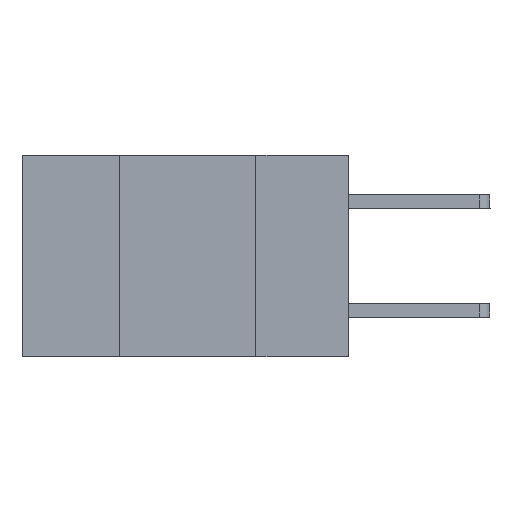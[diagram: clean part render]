
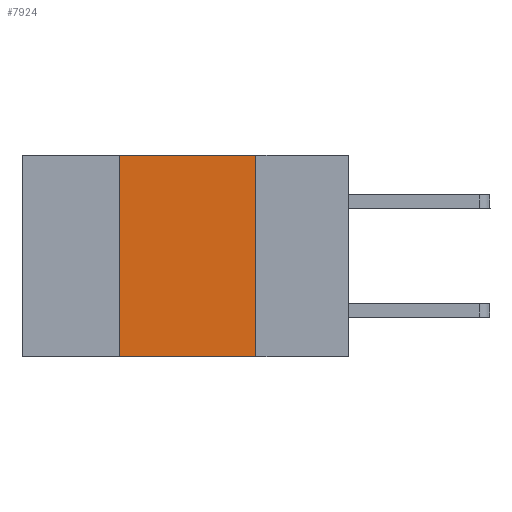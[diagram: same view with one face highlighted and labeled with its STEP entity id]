
A CAD part, left-side view. The second image highlights one B-rep face of the part: STEP entity #7924.
In plain terms, the highlighted planar face has unit normal (-1, 0, 0).
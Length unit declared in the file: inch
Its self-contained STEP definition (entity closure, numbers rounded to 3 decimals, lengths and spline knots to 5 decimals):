
#301 = DIRECTION ( 'NONE',  ( 1., 0., 0. ) ) ;
#354 = VERTEX_POINT ( 'NONE', #8715 ) ;
#697 = CARTESIAN_POINT ( 'NONE',  ( 0., 0.42, 0. ) ) ;
#1254 = PLANE ( 'NONE',  #8034 ) ;
#1422 = EDGE_CURVE ( 'NONE', #5762, #354, #6210, .T. ) ;
#1621 = EDGE_CURVE ( 'NONE', #354, #4686, #5054, .T. ) ;
#1622 = EDGE_CURVE ( 'NONE', #3400, #5762, #7652, .T. ) ;
#1808 = CARTESIAN_POINT ( 'NONE',  ( 0., 0.42, -0.37 ) ) ;
#1980 = CARTESIAN_POINT ( 'NONE',  ( 0., 0.17, -0.37 ) ) ;
#2040 = CARTESIAN_POINT ( 'NONE',  ( 0., 0.42, -0.37 ) ) ;
#2447 = DIRECTION ( 'NONE',  ( 0., -1., 0. ) ) ;
#2830 = VECTOR ( 'NONE', #9318, 39.37008 ) ;
#3367 = DIRECTION ( 'NONE',  ( 0., -1., 0. ) ) ;
#3400 = VERTEX_POINT ( 'NONE', #1808 ) ;
#4135 = VECTOR ( 'NONE', #6768, 39.37008 ) ;
#4367 = ORIENTED_EDGE ( 'NONE', *, *, #1422, .F. ) ;
#4686 = VERTEX_POINT ( 'NONE', #9959 ) ;
#4748 = EDGE_LOOP ( 'NONE', ( #9865, #4367, #9380, #6096 ) ) ;
#5054 = LINE ( 'NONE', #1980, #2830 ) ;
#5762 = VERTEX_POINT ( 'NONE', #697 ) ;
#5933 = FACE_OUTER_BOUND ( 'NONE', #4748, .T. ) ;
#6096 = ORIENTED_EDGE ( 'NONE', *, *, #7256, .T. ) ;
#6210 = LINE ( 'NONE', #6365, #8128 ) ;
#6365 = CARTESIAN_POINT ( 'NONE',  ( 0., 0.6, 0. ) ) ;
#6768 = DIRECTION ( 'NONE',  ( 0., 0., 1. ) ) ;
#7104 = CARTESIAN_POINT ( 'NONE',  ( 0., 0.6, -0.37 ) ) ;
#7256 = EDGE_CURVE ( 'NONE', #3400, #4686, #8100, .T. ) ;
#7652 = LINE ( 'NONE', #2040, #4135 ) ;
#7784 = VECTOR ( 'NONE', #3367, 39.37008 ) ;
#7924 = ADVANCED_FACE ( 'NONE', ( #5933 ), #1254, .F. ) ;
#8034 = AXIS2_PLACEMENT_3D ( 'NONE', #8447, #301, #9173 ) ;
#8100 = LINE ( 'NONE', #7104, #7784 ) ;
#8128 = VECTOR ( 'NONE', #2447, 39.37008 ) ;
#8447 = CARTESIAN_POINT ( 'NONE',  ( 0., 0.6, 0. ) ) ;
#8715 = CARTESIAN_POINT ( 'NONE',  ( 0., 0.17, 0. ) ) ;
#9173 = DIRECTION ( 'NONE',  ( 0., 0., -1. ) ) ;
#9318 = DIRECTION ( 'NONE',  ( 0., 0., -1. ) ) ;
#9380 = ORIENTED_EDGE ( 'NONE', *, *, #1622, .F. ) ;
#9865 = ORIENTED_EDGE ( 'NONE', *, *, #1621, .F. ) ;
#9959 = CARTESIAN_POINT ( 'NONE',  ( 0., 0.17, -0.37 ) ) ;
